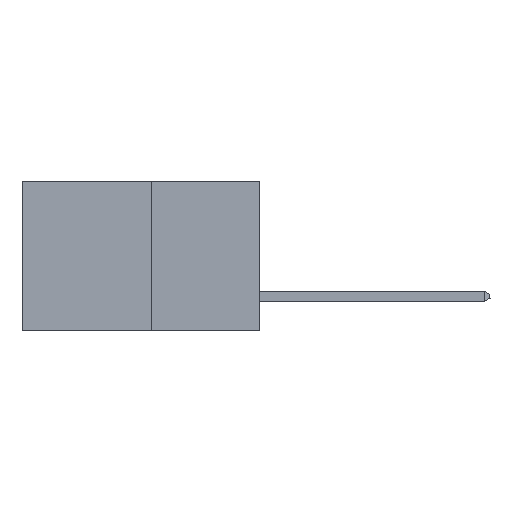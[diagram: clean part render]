
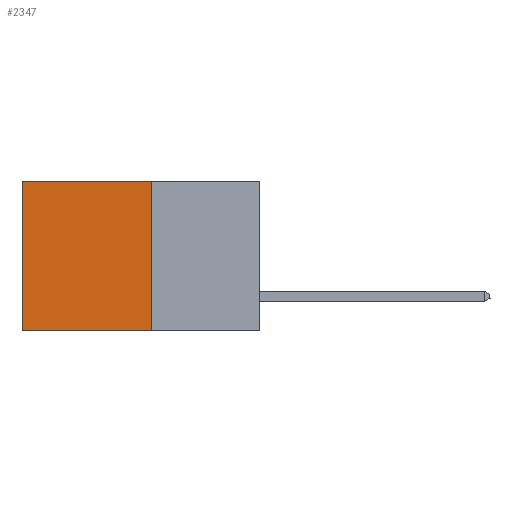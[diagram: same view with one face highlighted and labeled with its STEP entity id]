
A CAD part, left-side view. The second image highlights one B-rep face of the part: STEP entity #2347.
In plain terms, the highlighted planar face has unit normal (-1, 0, 0).
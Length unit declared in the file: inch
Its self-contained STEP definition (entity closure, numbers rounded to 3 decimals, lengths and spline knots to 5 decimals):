
#619 = DIRECTION ( 'NONE',  ( 0., 0., -1. ) ) ;
#671 = DIRECTION ( 'NONE',  ( 1., 0., 0. ) ) ;
#779 = PLANE ( 'NONE',  #16192 ) ;
#792 = VECTOR ( 'NONE', #2719, 39.37008 ) ;
#1249 = CARTESIAN_POINT ( 'NONE',  ( 0.277, 0.27, -0.37 ) ) ;
#1543 = LINE ( 'NONE', #16237, #4690 ) ;
#1983 = ORIENTED_EDGE ( 'NONE', *, *, #15535, .F. ) ;
#2292 = EDGE_CURVE ( 'NONE', #9578, #2668, #8012, .T. ) ;
#2347 = ADVANCED_FACE ( 'NONE', ( #10584 ), #779, .F. ) ;
#2426 = CARTESIAN_POINT ( 'NONE',  ( 0.277, 0.27, 0. ) ) ;
#2668 = VERTEX_POINT ( 'NONE', #11896 ) ;
#2719 = DIRECTION ( 'NONE',  ( 0., 1., 0. ) ) ;
#3240 = VERTEX_POINT ( 'NONE', #14308 ) ;
#3728 = ORIENTED_EDGE ( 'NONE', *, *, #15760, .T. ) ;
#3790 = DIRECTION ( 'NONE',  ( 0., 0., -1. ) ) ;
#4690 = VECTOR ( 'NONE', #7636, 39.37008 ) ;
#5090 = VECTOR ( 'NONE', #7396, 39.37008 ) ;
#5294 = VECTOR ( 'NONE', #3790, 39.37008 ) ;
#5712 = ORIENTED_EDGE ( 'NONE', *, *, #14667, .F. ) ;
#6040 = CARTESIAN_POINT ( 'NONE',  ( 0.277, 0.27, -0.37 ) ) ;
#7396 = DIRECTION ( 'NONE',  ( 0., 0., -1. ) ) ;
#7636 = DIRECTION ( 'NONE',  ( 0., 1., 0. ) ) ;
#8012 = LINE ( 'NONE', #2426, #792 ) ;
#9578 = VERTEX_POINT ( 'NONE', #12533 ) ;
#10249 = ORIENTED_EDGE ( 'NONE', *, *, #2292, .T. ) ;
#10584 = FACE_OUTER_BOUND ( 'NONE', #14094, .T. ) ;
#11896 = CARTESIAN_POINT ( 'NONE',  ( 0.277, 0.59, 0. ) ) ;
#12191 = LINE ( 'NONE', #15198, #5294 ) ;
#12533 = CARTESIAN_POINT ( 'NONE',  ( 0.277, 0.27, 0. ) ) ;
#14094 = EDGE_LOOP ( 'NONE', ( #3728, #5712, #1983, #10249 ) ) ;
#14308 = CARTESIAN_POINT ( 'NONE',  ( 0.277, 0.59, -0.37 ) ) ;
#14667 = EDGE_CURVE ( 'NONE', #16368, #3240, #1543, .T. ) ;
#14973 = CARTESIAN_POINT ( 'NONE',  ( 0.277, 0.27, -0.37 ) ) ;
#15191 = LINE ( 'NONE', #6040, #5090 ) ;
#15198 = CARTESIAN_POINT ( 'NONE',  ( 0.277, 0.59, -0.37 ) ) ;
#15535 = EDGE_CURVE ( 'NONE', #9578, #16368, #15191, .T. ) ;
#15760 = EDGE_CURVE ( 'NONE', #2668, #3240, #12191, .T. ) ;
#16192 = AXIS2_PLACEMENT_3D ( 'NONE', #1249, #671, #619 ) ;
#16237 = CARTESIAN_POINT ( 'NONE',  ( 0.277, 0.27, -0.37 ) ) ;
#16368 = VERTEX_POINT ( 'NONE', #14973 ) ;
